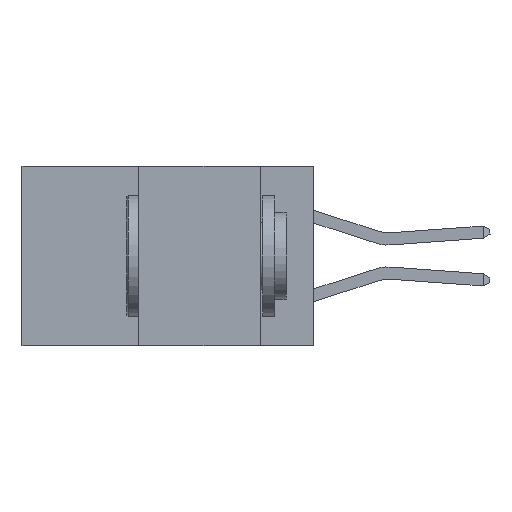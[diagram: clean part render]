
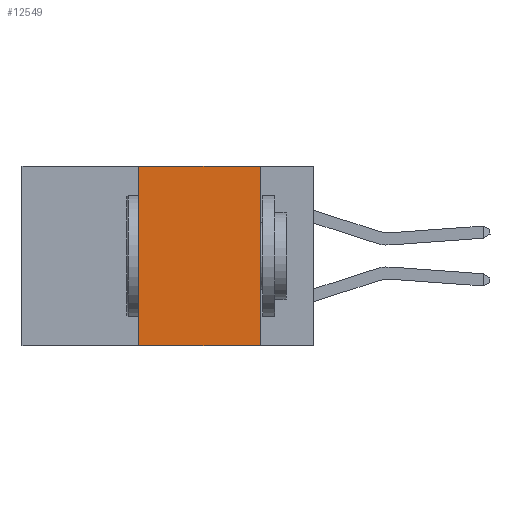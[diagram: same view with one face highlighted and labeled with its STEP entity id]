
A CAD part, left-side view. The second image highlights one B-rep face of the part: STEP entity #12549.
In plain terms, the highlighted planar face has unit normal (-1, 0, 0).
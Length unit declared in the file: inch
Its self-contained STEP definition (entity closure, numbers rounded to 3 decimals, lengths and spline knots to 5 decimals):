
#370 = VERTEX_POINT ( 'NONE', #19376 ) ;
#743 = ORIENTED_EDGE ( 'NONE', *, *, #2168, .F. ) ;
#2168 = EDGE_CURVE ( 'NONE', #13408, #25053, #23695, .T. ) ;
#3270 = PLANE ( 'NONE',  #10764 ) ;
#8079 = CARTESIAN_POINT ( 'NONE',  ( 0., 0.11, 0. ) ) ;
#9350 = CARTESIAN_POINT ( 'NONE',  ( 0., 0.6, 0. ) ) ;
#9642 = ORIENTED_EDGE ( 'NONE', *, *, #16311, .T. ) ;
#9896 = EDGE_LOOP ( 'NONE', ( #743, #15115, #29175, #9642 ) ) ;
#9918 = FACE_OUTER_BOUND ( 'NONE', #9896, .T. ) ;
#10764 = AXIS2_PLACEMENT_3D ( 'NONE', #11456, #14153, #32607 ) ;
#10808 = LINE ( 'NONE', #9350, #17909 ) ;
#11122 = LINE ( 'NONE', #18624, #18224 ) ;
#11456 = CARTESIAN_POINT ( 'NONE',  ( 0., 0.6, 0. ) ) ;
#12549 = ADVANCED_FACE ( 'NONE', ( #9918 ), #3270, .F. ) ;
#13375 = DIRECTION ( 'NONE',  ( 0., -1., 0. ) ) ;
#13408 = VERTEX_POINT ( 'NONE', #17245 ) ;
#14002 = EDGE_CURVE ( 'NONE', #370, #13408, #10808, .T. ) ;
#14153 = DIRECTION ( 'NONE',  ( 1., 0., 0. ) ) ;
#15115 = ORIENTED_EDGE ( 'NONE', *, *, #14002, .F. ) ;
#16311 = EDGE_CURVE ( 'NONE', #24509, #25053, #11122, .T. ) ;
#17245 = CARTESIAN_POINT ( 'NONE',  ( 0., 0.11, 0. ) ) ;
#17573 = CARTESIAN_POINT ( 'NONE',  ( 0., 0.36, 0. ) ) ;
#17909 = VECTOR ( 'NONE', #22613, 39.37008 ) ;
#17932 = LINE ( 'NONE', #17573, #31955 ) ;
#18224 = VECTOR ( 'NONE', #13375, 39.37008 ) ;
#18624 = CARTESIAN_POINT ( 'NONE',  ( 0., 0.6, -0.37 ) ) ;
#19376 = CARTESIAN_POINT ( 'NONE',  ( 0., 0.36, 0. ) ) ;
#20068 = CARTESIAN_POINT ( 'NONE',  ( 0., 0.36, -0.37 ) ) ;
#22613 = DIRECTION ( 'NONE',  ( 0., -1., 0. ) ) ;
#22795 = CARTESIAN_POINT ( 'NONE',  ( 0., 0.11, -0.37 ) ) ;
#23695 = LINE ( 'NONE', #8079, #30732 ) ;
#24509 = VERTEX_POINT ( 'NONE', #20068 ) ;
#25053 = VERTEX_POINT ( 'NONE', #22795 ) ;
#26702 = DIRECTION ( 'NONE',  ( 0., 0., -1. ) ) ;
#28699 = EDGE_CURVE ( 'NONE', #24509, #370, #17932, .T. ) ;
#29175 = ORIENTED_EDGE ( 'NONE', *, *, #28699, .F. ) ;
#30732 = VECTOR ( 'NONE', #26702, 39.37008 ) ;
#31955 = VECTOR ( 'NONE', #33342, 39.37008 ) ;
#32607 = DIRECTION ( 'NONE',  ( 0., 0., -1. ) ) ;
#33342 = DIRECTION ( 'NONE',  ( 0., 0., 1. ) ) ;
